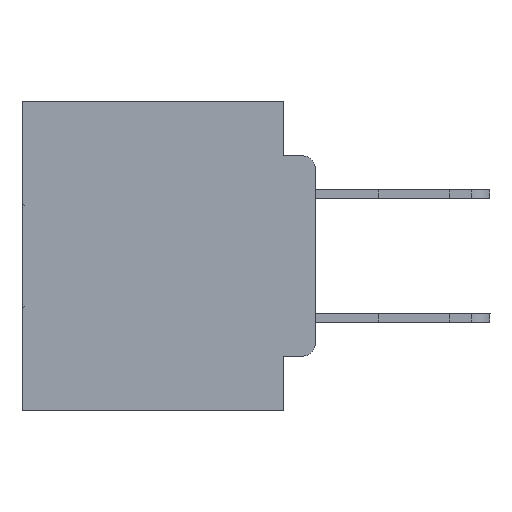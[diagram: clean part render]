
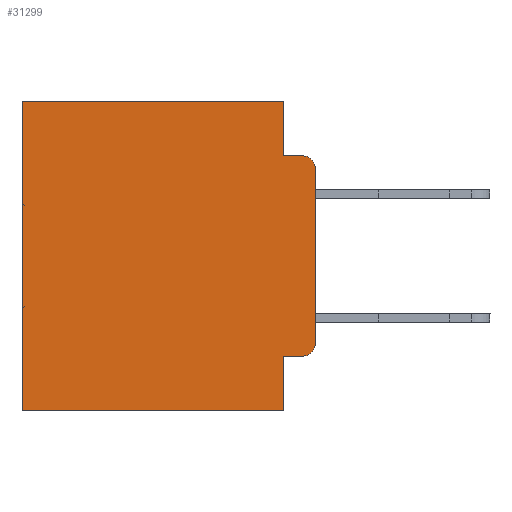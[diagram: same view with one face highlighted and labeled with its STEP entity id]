
A CAD part, left-side view. The second image highlights one B-rep face of the part: STEP entity #31299.
In plain terms, the highlighted planar face has unit normal (-1, 0, 0).
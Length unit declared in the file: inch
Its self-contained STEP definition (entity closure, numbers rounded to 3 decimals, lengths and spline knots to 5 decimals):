
#296 = VERTEX_POINT ( 'NONE', #15018 ) ;
#321 = EDGE_CURVE ( 'NONE', #23779, #30237, #30273, .T. ) ;
#376 = CARTESIAN_POINT ( 'NONE',  ( 0.298, 0.473, -0.5 ) ) ;
#463 = ORIENTED_EDGE ( 'NONE', *, *, #13280, .F. ) ;
#1002 = DIRECTION ( 'NONE',  ( 0., 0., -1. ) ) ;
#1308 = EDGE_CURVE ( 'NONE', #296, #23779, #14664, .T. ) ;
#2205 = LINE ( 'NONE', #5811, #32186 ) ;
#2518 = CARTESIAN_POINT ( 'NONE',  ( 0.298, 0.02, -0.0885 ) ) ;
#3087 = CARTESIAN_POINT ( 'NONE',  ( 0.298, 0.051, 0. ) ) ;
#3627 = VECTOR ( 'NONE', #22753, 39.37008 ) ;
#4085 = DIRECTION ( 'NONE',  ( -1., 0., 0. ) ) ;
#4174 = ORIENTED_EDGE ( 'NONE', *, *, #6998, .F. ) ;
#5479 = CARTESIAN_POINT ( 'NONE',  ( 0.298, 0.051, -0.4115 ) ) ;
#5620 = ORIENTED_EDGE ( 'NONE', *, *, #321, .T. ) ;
#5811 = CARTESIAN_POINT ( 'NONE',  ( 0.298, 0.051, -0.0885 ) ) ;
#6998 = EDGE_CURVE ( 'NONE', #33799, #10828, #18084, .T. ) ;
#7423 = VERTEX_POINT ( 'NONE', #20276 ) ;
#7471 = DIRECTION ( 'NONE',  ( 0., -1., 0. ) ) ;
#7698 = DIRECTION ( 'NONE',  ( 1., 0., 0. ) ) ;
#7899 = AXIS2_PLACEMENT_3D ( 'NONE', #18124, #7698, #10247 ) ;
#8577 = DIRECTION ( 'NONE',  ( 0., 0., -1. ) ) ;
#8641 = VERTEX_POINT ( 'NONE', #30832 ) ;
#9470 = VECTOR ( 'NONE', #8577, 39.37008 ) ;
#9854 = EDGE_LOOP ( 'NONE', ( #26506, #25785, #25955, #463, #26947, #5620, #33794, #4174, #22549, #27872 ) ) ;
#9946 = CARTESIAN_POINT ( 'NONE',  ( 0.298, 0.473, 0. ) ) ;
#10247 = DIRECTION ( 'NONE',  ( 0., 0., -1. ) ) ;
#10828 = VERTEX_POINT ( 'NONE', #12602 ) ;
#11130 = VECTOR ( 'NONE', #25618, 39.37008 ) ;
#11340 = DIRECTION ( 'NONE',  ( 0., -1., 0. ) ) ;
#11653 = LINE ( 'NONE', #20274, #23884 ) ;
#12602 = CARTESIAN_POINT ( 'NONE',  ( 0.298, 0.051, -0.5 ) ) ;
#12805 = PLANE ( 'NONE',  #7899 ) ;
#13280 = EDGE_CURVE ( 'NONE', #296, #19364, #24371, .T. ) ;
#13378 = VECTOR ( 'NONE', #1002, 39.37008 ) ;
#13804 = EDGE_CURVE ( 'NONE', #19364, #29450, #2205, .T. ) ;
#14111 = AXIS2_PLACEMENT_3D ( 'NONE', #17661, #15083, #28312 ) ;
#14664 = LINE ( 'NONE', #15714, #15481 ) ;
#14774 = CARTESIAN_POINT ( 'NONE',  ( 0.298, 0.051, -0.0885 ) ) ;
#14922 = DIRECTION ( 'NONE',  ( 0., 0., -1. ) ) ;
#15018 = CARTESIAN_POINT ( 'NONE',  ( 0.298, 0.051, 0. ) ) ;
#15083 = DIRECTION ( 'NONE',  ( -1., 0., 0. ) ) ;
#15129 = CARTESIAN_POINT ( 'NONE',  ( 0.298, 0., -0.3915 ) ) ;
#15415 = CARTESIAN_POINT ( 'NONE',  ( 0.298, 0.051, -0.4115 ) ) ;
#15481 = VECTOR ( 'NONE', #28402, 39.37008 ) ;
#15714 = CARTESIAN_POINT ( 'NONE',  ( 0.298, 0., 0. ) ) ;
#17151 = CARTESIAN_POINT ( 'NONE',  ( 0.298, 0.02, -0.3915 ) ) ;
#17661 = CARTESIAN_POINT ( 'NONE',  ( 0.298, 0.02, -0.1085 ) ) ;
#18036 = VECTOR ( 'NONE', #7471, 39.37008 ) ;
#18084 = LINE ( 'NONE', #21206, #9470 ) ;
#18124 = CARTESIAN_POINT ( 'NONE',  ( 0.298, 0., 0. ) ) ;
#19364 = VERTEX_POINT ( 'NONE', #14774 ) ;
#19781 = CIRCLE ( 'NONE', #22391, 0.02 ) ;
#20274 = CARTESIAN_POINT ( 'NONE',  ( 0.298, 0., 0. ) ) ;
#20276 = CARTESIAN_POINT ( 'NONE',  ( 0.298, 0., -0.1085 ) ) ;
#20288 = CARTESIAN_POINT ( 'NONE',  ( 0.298, 0.473, 0. ) ) ;
#20709 = EDGE_CURVE ( 'NONE', #7423, #28098, #11653, .T. ) ;
#21152 = EDGE_CURVE ( 'NONE', #8641, #28098, #19781, .T. ) ;
#21206 = CARTESIAN_POINT ( 'NONE',  ( 0.298, 0.051, 0. ) ) ;
#21963 = EDGE_CURVE ( 'NONE', #7423, #29450, #22960, .T. ) ;
#22391 = AXIS2_PLACEMENT_3D ( 'NONE', #17151, #4085, #24690 ) ;
#22549 = ORIENTED_EDGE ( 'NONE', *, *, #33009, .T. ) ;
#22753 = DIRECTION ( 'NONE',  ( 0., 0., -1. ) ) ;
#22960 = CIRCLE ( 'NONE', #14111, 0.02 ) ;
#23779 = VERTEX_POINT ( 'NONE', #20288 ) ;
#23884 = VECTOR ( 'NONE', #14922, 39.37008 ) ;
#24371 = LINE ( 'NONE', #3087, #13378 ) ;
#24690 = DIRECTION ( 'NONE',  ( 0., 0., -1. ) ) ;
#25499 = CARTESIAN_POINT ( 'NONE',  ( 0.298, 0., -0.5 ) ) ;
#25618 = DIRECTION ( 'NONE',  ( 0., 1., 0. ) ) ;
#25785 = ORIENTED_EDGE ( 'NONE', *, *, #21963, .T. ) ;
#25955 = ORIENTED_EDGE ( 'NONE', *, *, #13804, .F. ) ;
#26284 = LINE ( 'NONE', #25499, #11130 ) ;
#26341 = FACE_OUTER_BOUND ( 'NONE', #9854, .T. ) ;
#26506 = ORIENTED_EDGE ( 'NONE', *, *, #20709, .F. ) ;
#26947 = ORIENTED_EDGE ( 'NONE', *, *, #1308, .T. ) ;
#27044 = LINE ( 'NONE', #15415, #18036 ) ;
#27872 = ORIENTED_EDGE ( 'NONE', *, *, #21152, .T. ) ;
#28098 = VERTEX_POINT ( 'NONE', #15129 ) ;
#28312 = DIRECTION ( 'NONE',  ( 0., 0., -1. ) ) ;
#28402 = DIRECTION ( 'NONE',  ( 0., 1., 0. ) ) ;
#29450 = VERTEX_POINT ( 'NONE', #2518 ) ;
#30237 = VERTEX_POINT ( 'NONE', #376 ) ;
#30273 = LINE ( 'NONE', #9946, #3627 ) ;
#30832 = CARTESIAN_POINT ( 'NONE',  ( 0.298, 0.02, -0.4115 ) ) ;
#31299 = ADVANCED_FACE ( 'NONE', ( #26341 ), #12805, .F. ) ;
#32186 = VECTOR ( 'NONE', #11340, 39.37008 ) ;
#32294 = EDGE_CURVE ( 'NONE', #10828, #30237, #26284, .T. ) ;
#33009 = EDGE_CURVE ( 'NONE', #33799, #8641, #27044, .T. ) ;
#33794 = ORIENTED_EDGE ( 'NONE', *, *, #32294, .F. ) ;
#33799 = VERTEX_POINT ( 'NONE', #5479 ) ;
